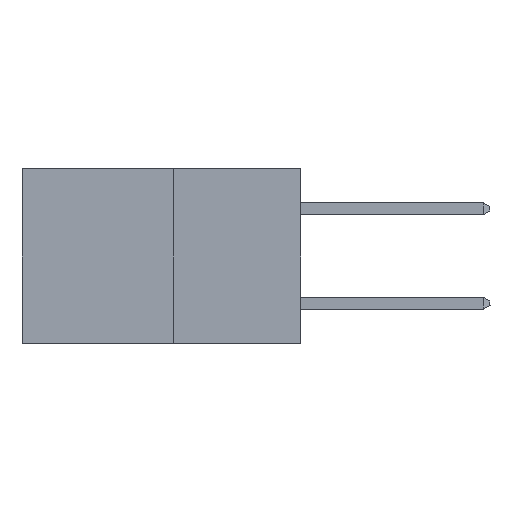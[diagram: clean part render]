
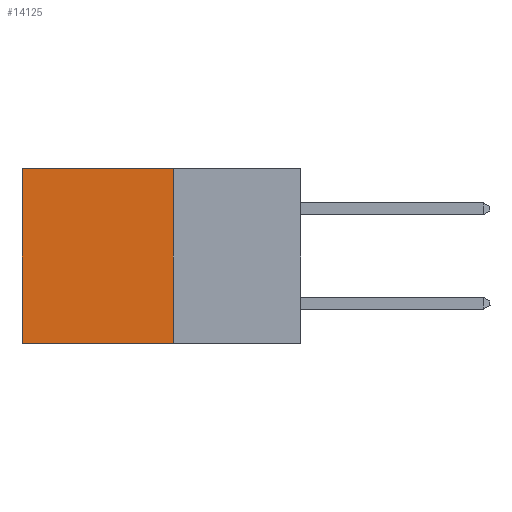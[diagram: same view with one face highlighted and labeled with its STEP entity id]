
A CAD part, left-side view. The second image highlights one B-rep face of the part: STEP entity #14125.
In plain terms, the highlighted planar face has unit normal (-1, 0, 0).
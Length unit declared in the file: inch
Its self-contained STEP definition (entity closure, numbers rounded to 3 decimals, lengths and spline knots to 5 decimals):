
#160 = VERTEX_POINT ( 'NONE', #205 ) ;
#196 = ORIENTED_EDGE ( 'NONE', *, *, #6378, .T. ) ;
#205 = CARTESIAN_POINT ( 'NONE',  ( 0.277, 0.59, 0. ) ) ;
#492 = ORIENTED_EDGE ( 'NONE', *, *, #12060, .F. ) ;
#1653 = CARTESIAN_POINT ( 'NONE',  ( 0.277, 0.59, -0.37 ) ) ;
#2809 = DIRECTION ( 'NONE',  ( 0., 0., -1. ) ) ;
#3902 = CARTESIAN_POINT ( 'NONE',  ( 0.277, 0.27, 0. ) ) ;
#5091 = VERTEX_POINT ( 'NONE', #21167 ) ;
#5730 = CARTESIAN_POINT ( 'NONE',  ( 0.277, 0.27, -0.37 ) ) ;
#5772 = VECTOR ( 'NONE', #2809, 39.37008 ) ;
#6378 = EDGE_CURVE ( 'NONE', #160, #5091, #7337, .T. ) ;
#6629 = DIRECTION ( 'NONE',  ( 0., 0., -1. ) ) ;
#7337 = LINE ( 'NONE', #1653, #5772 ) ;
#9455 = CARTESIAN_POINT ( 'NONE',  ( 0.277, 0.27, -0.37 ) ) ;
#11181 = CARTESIAN_POINT ( 'NONE',  ( 0.277, 0.27, 0. ) ) ;
#12060 = EDGE_CURVE ( 'NONE', #17121, #26599, #17826, .T. ) ;
#12689 = EDGE_CURVE ( 'NONE', #17121, #160, #21889, .T. ) ;
#14094 = VECTOR ( 'NONE', #27871, 39.37008 ) ;
#14125 = ADVANCED_FACE ( 'NONE', ( #17337 ), #16229, .F. ) ;
#15566 = EDGE_CURVE ( 'NONE', #26599, #5091, #20266, .T. ) ;
#16229 = PLANE ( 'NONE',  #23163 ) ;
#17121 = VERTEX_POINT ( 'NONE', #11181 ) ;
#17337 = FACE_OUTER_BOUND ( 'NONE', #28785, .T. ) ;
#17739 = DIRECTION ( 'NONE',  ( 0., 0., -1. ) ) ;
#17826 = LINE ( 'NONE', #5730, #24137 ) ;
#20026 = ORIENTED_EDGE ( 'NONE', *, *, #12689, .T. ) ;
#20266 = LINE ( 'NONE', #9455, #25811 ) ;
#20975 = DIRECTION ( 'NONE',  ( 1., 0., 0. ) ) ;
#21109 = CARTESIAN_POINT ( 'NONE',  ( 0.277, 0.27, -0.37 ) ) ;
#21167 = CARTESIAN_POINT ( 'NONE',  ( 0.277, 0.59, -0.37 ) ) ;
#21889 = LINE ( 'NONE', #3902, #14094 ) ;
#23163 = AXIS2_PLACEMENT_3D ( 'NONE', #25625, #20975, #6629 ) ;
#24137 = VECTOR ( 'NONE', #17739, 39.37008 ) ;
#25625 = CARTESIAN_POINT ( 'NONE',  ( 0.277, 0.27, -0.37 ) ) ;
#25811 = VECTOR ( 'NONE', #28467, 39.37008 ) ;
#26599 = VERTEX_POINT ( 'NONE', #21109 ) ;
#27612 = ORIENTED_EDGE ( 'NONE', *, *, #15566, .F. ) ;
#27871 = DIRECTION ( 'NONE',  ( 0., 1., 0. ) ) ;
#28467 = DIRECTION ( 'NONE',  ( 0., 1., 0. ) ) ;
#28785 = EDGE_LOOP ( 'NONE', ( #196, #27612, #492, #20026 ) ) ;
